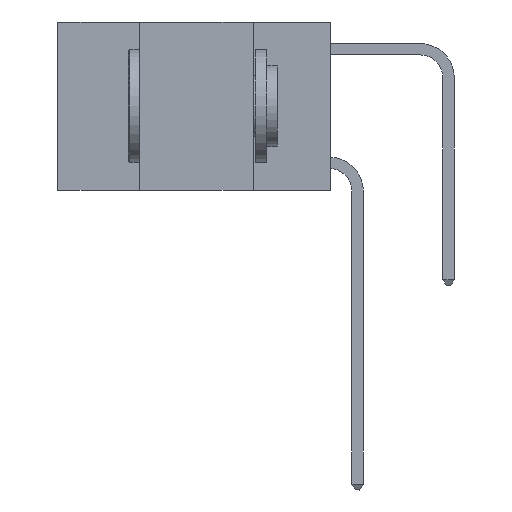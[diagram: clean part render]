
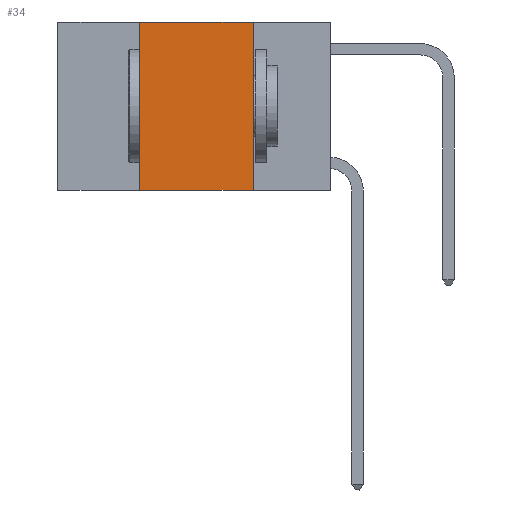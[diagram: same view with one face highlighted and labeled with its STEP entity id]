
A CAD part, left-side view. The second image highlights one B-rep face of the part: STEP entity #34.
In plain terms, the highlighted planar face has unit normal (-1, 0, 0).
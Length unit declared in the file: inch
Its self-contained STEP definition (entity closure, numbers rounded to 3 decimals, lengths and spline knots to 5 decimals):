
#34 = ADVANCED_FACE ( 'NONE', ( #11554 ), #12969, .F. ) ;
#2670 = CARTESIAN_POINT ( 'NONE',  ( 0., 0.6, -0.37 ) ) ;
#2809 = VERTEX_POINT ( 'NONE', #31566 ) ;
#3018 = VECTOR ( 'NONE', #32757, 39.37008 ) ;
#3985 = EDGE_CURVE ( 'NONE', #15217, #2809, #4755, .T. ) ;
#4122 = VERTEX_POINT ( 'NONE', #26383 ) ;
#4595 = CARTESIAN_POINT ( 'NONE',  ( 0., 0.42, 0. ) ) ;
#4755 = LINE ( 'NONE', #2670, #17812 ) ;
#5302 = EDGE_CURVE ( 'NONE', #27764, #4122, #10090, .T. ) ;
#6210 = CARTESIAN_POINT ( 'NONE',  ( 0., 0.42, -0.37 ) ) ;
#6512 = DIRECTION ( 'NONE',  ( 0., -1., 0. ) ) ;
#7151 = ORIENTED_EDGE ( 'NONE', *, *, #14664, .F. ) ;
#8203 = AXIS2_PLACEMENT_3D ( 'NONE', #24395, #21404, #25528 ) ;
#10090 = LINE ( 'NONE', #24736, #30740 ) ;
#10951 = ORIENTED_EDGE ( 'NONE', *, *, #5302, .F. ) ;
#11554 = FACE_OUTER_BOUND ( 'NONE', #25004, .T. ) ;
#12043 = LINE ( 'NONE', #4595, #19756 ) ;
#12449 = DIRECTION ( 'NONE',  ( 0., 0., 1. ) ) ;
#12969 = PLANE ( 'NONE',  #8203 ) ;
#14664 = EDGE_CURVE ( 'NONE', #4122, #2809, #22921, .T. ) ;
#15217 = VERTEX_POINT ( 'NONE', #6210 ) ;
#15526 = ORIENTED_EDGE ( 'NONE', *, *, #3985, .T. ) ;
#17812 = VECTOR ( 'NONE', #23437, 39.37008 ) ;
#19718 = ORIENTED_EDGE ( 'NONE', *, *, #28987, .F. ) ;
#19756 = VECTOR ( 'NONE', #12449, 39.37008 ) ;
#21404 = DIRECTION ( 'NONE',  ( 1., 0., 0. ) ) ;
#22921 = LINE ( 'NONE', #30136, #3018 ) ;
#23437 = DIRECTION ( 'NONE',  ( 0., -1., 0. ) ) ;
#24395 = CARTESIAN_POINT ( 'NONE',  ( 0., 0.6, 0. ) ) ;
#24736 = CARTESIAN_POINT ( 'NONE',  ( 0., 0.6, 0. ) ) ;
#25004 = EDGE_LOOP ( 'NONE', ( #7151, #10951, #19718, #15526 ) ) ;
#25528 = DIRECTION ( 'NONE',  ( 0., 0., -1. ) ) ;
#26383 = CARTESIAN_POINT ( 'NONE',  ( 0., 0.17, 0. ) ) ;
#27764 = VERTEX_POINT ( 'NONE', #30287 ) ;
#28987 = EDGE_CURVE ( 'NONE', #15217, #27764, #12043, .T. ) ;
#30136 = CARTESIAN_POINT ( 'NONE',  ( 0., 0.17, 0. ) ) ;
#30287 = CARTESIAN_POINT ( 'NONE',  ( 0., 0.42, 0. ) ) ;
#30740 = VECTOR ( 'NONE', #6512, 39.37008 ) ;
#31566 = CARTESIAN_POINT ( 'NONE',  ( 0., 0.17, -0.37 ) ) ;
#32757 = DIRECTION ( 'NONE',  ( 0., 0., -1. ) ) ;
